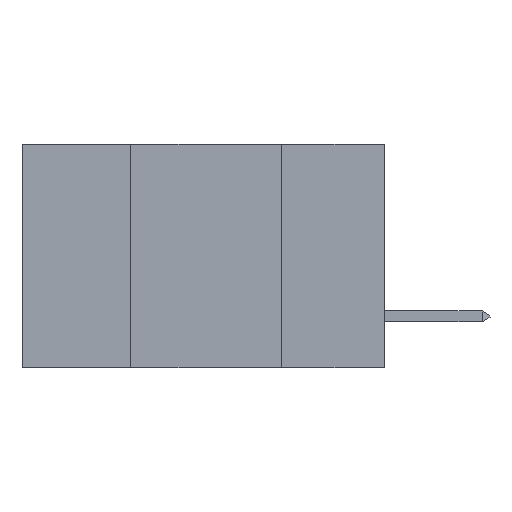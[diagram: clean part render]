
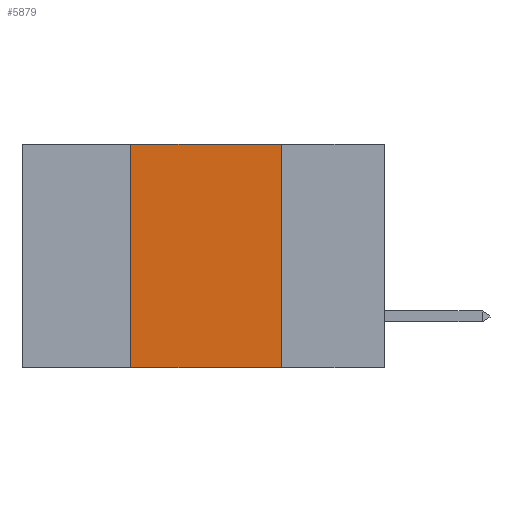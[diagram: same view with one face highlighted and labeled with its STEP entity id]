
A CAD part, left-side view. The second image highlights one B-rep face of the part: STEP entity #5879.
In plain terms, the highlighted planar face has unit normal (-1, 0, 0).
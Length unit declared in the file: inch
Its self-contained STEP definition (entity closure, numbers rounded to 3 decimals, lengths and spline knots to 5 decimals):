
#615 = EDGE_CURVE ( 'NONE', #8886, #7896, #3474, .T. ) ;
#981 = CARTESIAN_POINT ( 'NONE',  ( 0., 0.42, -0.37 ) ) ;
#2543 = EDGE_CURVE ( 'NONE', #5233, #7896, #12033, .T. ) ;
#3100 = DIRECTION ( 'NONE',  ( 0., 0., 1. ) ) ;
#3260 = EDGE_CURVE ( 'NONE', #3895, #8886, #4698, .T. ) ;
#3474 = LINE ( 'NONE', #13638, #7167 ) ;
#3756 = CARTESIAN_POINT ( 'NONE',  ( 0., 0.6, 0. ) ) ;
#3895 = VERTEX_POINT ( 'NONE', #8490 ) ;
#4212 = CARTESIAN_POINT ( 'NONE',  ( 0., 0.6, -0.37 ) ) ;
#4698 = LINE ( 'NONE', #8576, #11571 ) ;
#5136 = LINE ( 'NONE', #14032, #15096 ) ;
#5233 = VERTEX_POINT ( 'NONE', #981 ) ;
#5695 = CARTESIAN_POINT ( 'NONE',  ( 0., 0.17, 0. ) ) ;
#5879 = ADVANCED_FACE ( 'NONE', ( #12977 ), #13308, .F. ) ;
#6541 = DIRECTION ( 'NONE',  ( 0., 0., -1. ) ) ;
#6566 = EDGE_LOOP ( 'NONE', ( #8183, #8121, #8104, #8086 ) ) ;
#6860 = DIRECTION ( 'NONE',  ( 0., 0., -1. ) ) ;
#7167 = VECTOR ( 'NONE', #6860, 39.37008 ) ;
#7896 = VERTEX_POINT ( 'NONE', #17083 ) ;
#8086 = ORIENTED_EDGE ( 'NONE', *, *, #2543, .T. ) ;
#8104 = ORIENTED_EDGE ( 'NONE', *, *, #17334, .F. ) ;
#8121 = ORIENTED_EDGE ( 'NONE', *, *, #3260, .F. ) ;
#8183 = ORIENTED_EDGE ( 'NONE', *, *, #615, .F. ) ;
#8490 = CARTESIAN_POINT ( 'NONE',  ( 0., 0.42, 0. ) ) ;
#8576 = CARTESIAN_POINT ( 'NONE',  ( 0., 0.6, 0. ) ) ;
#8886 = VERTEX_POINT ( 'NONE', #5695 ) ;
#11571 = VECTOR ( 'NONE', #16543, 39.37008 ) ;
#11610 = VECTOR ( 'NONE', #17611, 39.37008 ) ;
#12033 = LINE ( 'NONE', #4212, #11610 ) ;
#12977 = FACE_OUTER_BOUND ( 'NONE', #6566, .T. ) ;
#13308 = PLANE ( 'NONE',  #13337 ) ;
#13337 = AXIS2_PLACEMENT_3D ( 'NONE', #3756, #14632, #6541 ) ;
#13638 = CARTESIAN_POINT ( 'NONE',  ( 0., 0.17, 0. ) ) ;
#14032 = CARTESIAN_POINT ( 'NONE',  ( 0., 0.42, 0. ) ) ;
#14632 = DIRECTION ( 'NONE',  ( 1., 0., 0. ) ) ;
#15096 = VECTOR ( 'NONE', #3100, 39.37008 ) ;
#16543 = DIRECTION ( 'NONE',  ( 0., -1., 0. ) ) ;
#17083 = CARTESIAN_POINT ( 'NONE',  ( 0., 0.17, -0.37 ) ) ;
#17334 = EDGE_CURVE ( 'NONE', #5233, #3895, #5136, .T. ) ;
#17611 = DIRECTION ( 'NONE',  ( 0., -1., 0. ) ) ;
